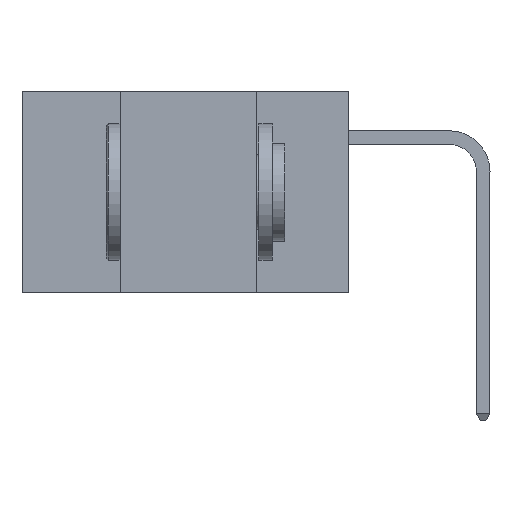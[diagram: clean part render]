
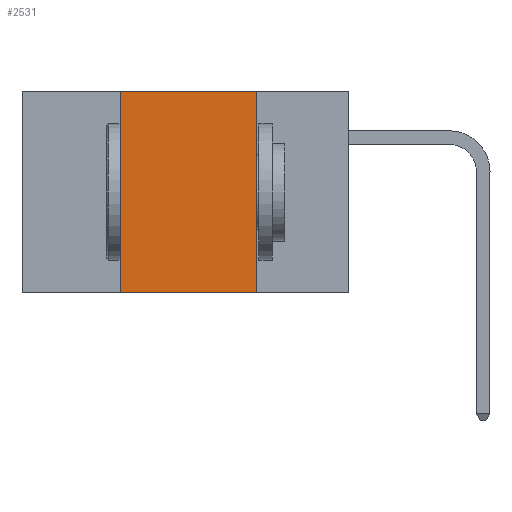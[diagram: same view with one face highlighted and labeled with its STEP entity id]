
A CAD part, left-side view. The second image highlights one B-rep face of the part: STEP entity #2531.
In plain terms, the highlighted planar face has unit normal (-1, 0, 0).
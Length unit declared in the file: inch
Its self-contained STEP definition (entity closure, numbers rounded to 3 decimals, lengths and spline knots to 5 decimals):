
#710 = VERTEX_POINT ( 'NONE', #10897 ) ;
#1066 = CARTESIAN_POINT ( 'NONE',  ( 0., 0.42, 0. ) ) ;
#2531 = ADVANCED_FACE ( 'NONE', ( #23636 ), #17992, .F. ) ;
#3662 = VERTEX_POINT ( 'NONE', #21649 ) ;
#3752 = VECTOR ( 'NONE', #9670, 39.37008 ) ;
#3779 = ORIENTED_EDGE ( 'NONE', *, *, #8685, .F. ) ;
#4943 = ORIENTED_EDGE ( 'NONE', *, *, #13556, .F. ) ;
#5376 = VERTEX_POINT ( 'NONE', #1066 ) ;
#5928 = CARTESIAN_POINT ( 'NONE',  ( 0., 0.17, 0. ) ) ;
#6780 = LINE ( 'NONE', #22740, #20833 ) ;
#8421 = EDGE_CURVE ( 'NONE', #10836, #3662, #6780, .T. ) ;
#8685 = EDGE_CURVE ( 'NONE', #710, #5376, #16844, .T. ) ;
#9416 = LINE ( 'NONE', #12855, #18651 ) ;
#9593 = EDGE_LOOP ( 'NONE', ( #21370, #4943, #3779, #15866 ) ) ;
#9670 = DIRECTION ( 'NONE',  ( 0., -1., 0. ) ) ;
#10836 = VERTEX_POINT ( 'NONE', #5928 ) ;
#10897 = CARTESIAN_POINT ( 'NONE',  ( 0., 0.42, -0.37 ) ) ;
#12575 = DIRECTION ( 'NONE',  ( 0., 0., 1. ) ) ;
#12855 = CARTESIAN_POINT ( 'NONE',  ( 0., 0.6, 0. ) ) ;
#13556 = EDGE_CURVE ( 'NONE', #5376, #10836, #9416, .T. ) ;
#14131 = LINE ( 'NONE', #22430, #3752 ) ;
#14732 = DIRECTION ( 'NONE',  ( 0., -1., 0. ) ) ;
#15108 = VECTOR ( 'NONE', #12575, 39.37008 ) ;
#15866 = ORIENTED_EDGE ( 'NONE', *, *, #16838, .T. ) ;
#15969 = AXIS2_PLACEMENT_3D ( 'NONE', #18123, #17336, #17121 ) ;
#16838 = EDGE_CURVE ( 'NONE', #710, #3662, #14131, .T. ) ;
#16844 = LINE ( 'NONE', #21723, #15108 ) ;
#17121 = DIRECTION ( 'NONE',  ( 0., 0., -1. ) ) ;
#17336 = DIRECTION ( 'NONE',  ( 1., 0., 0. ) ) ;
#17379 = DIRECTION ( 'NONE',  ( 0., 0., -1. ) ) ;
#17992 = PLANE ( 'NONE',  #15969 ) ;
#18123 = CARTESIAN_POINT ( 'NONE',  ( 0., 0.6, 0. ) ) ;
#18651 = VECTOR ( 'NONE', #14732, 39.37008 ) ;
#20833 = VECTOR ( 'NONE', #17379, 39.37008 ) ;
#21370 = ORIENTED_EDGE ( 'NONE', *, *, #8421, .F. ) ;
#21649 = CARTESIAN_POINT ( 'NONE',  ( 0., 0.17, -0.37 ) ) ;
#21723 = CARTESIAN_POINT ( 'NONE',  ( 0., 0.42, 0. ) ) ;
#22430 = CARTESIAN_POINT ( 'NONE',  ( 0., 0.6, -0.37 ) ) ;
#22740 = CARTESIAN_POINT ( 'NONE',  ( 0., 0.17, 0. ) ) ;
#23636 = FACE_OUTER_BOUND ( 'NONE', #9593, .T. ) ;
